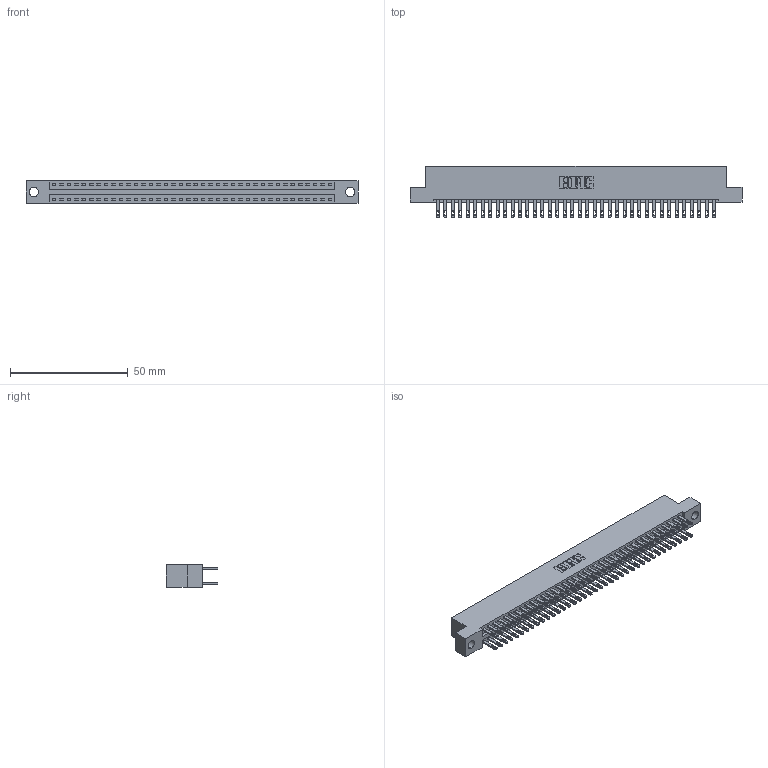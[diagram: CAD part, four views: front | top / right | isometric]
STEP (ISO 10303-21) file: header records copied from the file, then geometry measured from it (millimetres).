
FILE_DESCRIPTION (( 'STEP AP203' ), '1' );
FILE_NAME ('346-076-500-204.STEP', '2018-08-29T03:23:23', ( '' ), ( '' ), 'SwSTEP 2.0', 'SolidWorks 2016', '' );
FILE_SCHEMA (( 'CONFIG_CONTROL_DESIGN' ));
Length unit declared in the file: inch
Products named in the file (3): 345-292-001_345-293-100; 346-076-500-204; 346 Part_Flush Mounting Lugs - 0.156 Dia-TH
Assembly tree (77 placements, depth 2):
  346-076-500-204
    346 Part_Flush Mounting Lugs - 0.156 Dia-TH
    345-292-001_345-293-100  x76
Bounding box: 141.22 x 21.84 x 9.4 mm (x, y, z)
Volume: 13884.4 mm3; surface area: 19631 mm2
Topology: 77 solids, 77 shells, 3770 faces, 11501 edges, 7666 vertices
Faces by surface type: plane 2280, cylinder 1490
Entity records: 25271 total; most frequent: CARTESIAN_POINT 4168, ORIENTED_EDGE 4102, DIRECTION 3727, EDGE_CURVE 2051, VECTOR 1763, LINE 1763, VERTEX_POINT 1366, AXIS2_PLACEMENT_3D 982
